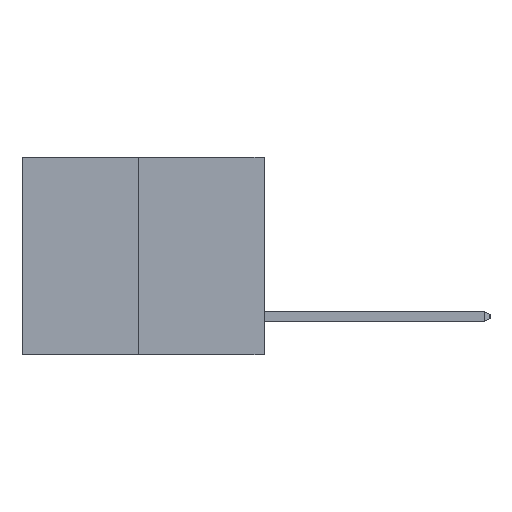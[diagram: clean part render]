
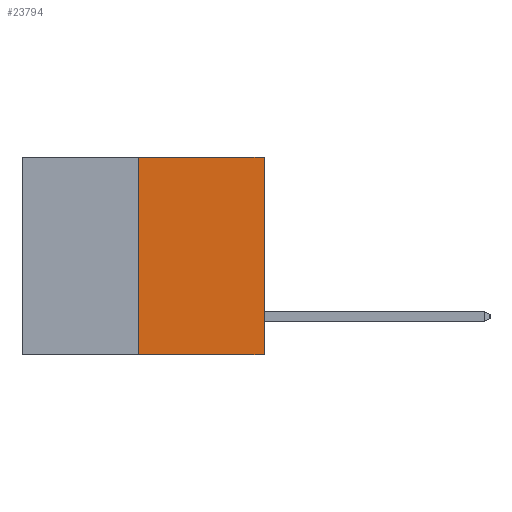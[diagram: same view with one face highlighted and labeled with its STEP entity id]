
A CAD part, left-side view. The second image highlights one B-rep face of the part: STEP entity #23794.
In plain terms, the highlighted planar face has unit normal (-1, 0, 0).
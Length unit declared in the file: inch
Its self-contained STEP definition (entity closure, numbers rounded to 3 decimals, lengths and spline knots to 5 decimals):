
#215 = VECTOR ( 'NONE', #2150, 39.37008 ) ;
#1339 = EDGE_CURVE ( 'NONE', #19332, #15134, #19681, .T. ) ;
#2150 = DIRECTION ( 'NONE',  ( 0., -1., 0. ) ) ;
#2392 = EDGE_CURVE ( 'NONE', #15877, #6568, #24203, .T. ) ;
#3239 = EDGE_CURVE ( 'NONE', #15877, #19332, #5428, .T. ) ;
#3414 = CARTESIAN_POINT ( 'NONE',  ( 0., 0., 0. ) ) ;
#5428 = LINE ( 'NONE', #13955, #215 ) ;
#6568 = VERTEX_POINT ( 'NONE', #10545 ) ;
#7034 = VECTOR ( 'NONE', #18667, 39.37008 ) ;
#7091 = CARTESIAN_POINT ( 'NONE',  ( 0., 0.312, -0.49 ) ) ;
#7283 = CARTESIAN_POINT ( 'NONE',  ( 0., 0.312, -0.49 ) ) ;
#8013 = VECTOR ( 'NONE', #21491, 39.37008 ) ;
#8064 = VECTOR ( 'NONE', #11436, 39.37008 ) ;
#8926 = DIRECTION ( 'NONE',  ( 1., 0., 0. ) ) ;
#9270 = ORIENTED_EDGE ( 'NONE', *, *, #3239, .T. ) ;
#9384 = CARTESIAN_POINT ( 'NONE',  ( 0., 0.6, 0. ) ) ;
#10545 = CARTESIAN_POINT ( 'NONE',  ( 0., 0.312, 0. ) ) ;
#10820 = LINE ( 'NONE', #9384, #8064 ) ;
#10823 = DIRECTION ( 'NONE',  ( 0., 0., -1. ) ) ;
#11436 = DIRECTION ( 'NONE',  ( 0., -1., 0. ) ) ;
#12760 = ORIENTED_EDGE ( 'NONE', *, *, #17511, .F. ) ;
#13955 = CARTESIAN_POINT ( 'NONE',  ( 0., 0.6, -0.49 ) ) ;
#15134 = VERTEX_POINT ( 'NONE', #3414 ) ;
#15877 = VERTEX_POINT ( 'NONE', #7283 ) ;
#17511 = EDGE_CURVE ( 'NONE', #6568, #15134, #10820, .T. ) ;
#18667 = DIRECTION ( 'NONE',  ( 0., 0., 1. ) ) ;
#19332 = VERTEX_POINT ( 'NONE', #22210 ) ;
#19538 = CARTESIAN_POINT ( 'NONE',  ( 0., 0., 0. ) ) ;
#19681 = LINE ( 'NONE', #19538, #8013 ) ;
#21128 = FACE_OUTER_BOUND ( 'NONE', #23394, .T. ) ;
#21491 = DIRECTION ( 'NONE',  ( 0., 0., 1. ) ) ;
#22210 = CARTESIAN_POINT ( 'NONE',  ( 0., 0., -0.49 ) ) ;
#22561 = PLANE ( 'NONE',  #24740 ) ;
#23394 = EDGE_LOOP ( 'NONE', ( #23661, #9270, #24982, #12760 ) ) ;
#23661 = ORIENTED_EDGE ( 'NONE', *, *, #2392, .F. ) ;
#23794 = ADVANCED_FACE ( 'NONE', ( #21128 ), #22561, .F. ) ;
#24203 = LINE ( 'NONE', #7091, #7034 ) ;
#24740 = AXIS2_PLACEMENT_3D ( 'NONE', #24784, #8926, #10823 ) ;
#24784 = CARTESIAN_POINT ( 'NONE',  ( 0., 0.6, 0. ) ) ;
#24982 = ORIENTED_EDGE ( 'NONE', *, *, #1339, .T. ) ;
